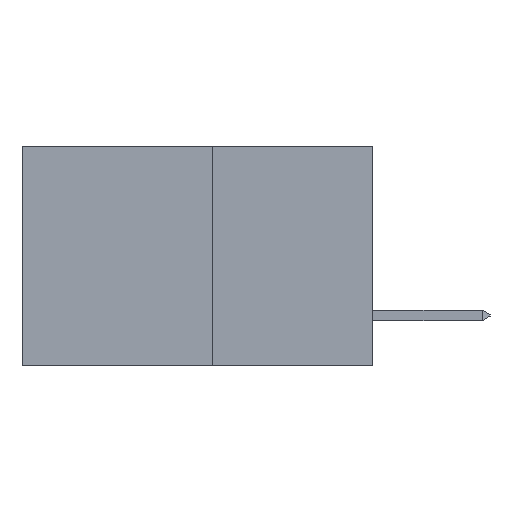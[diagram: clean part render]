
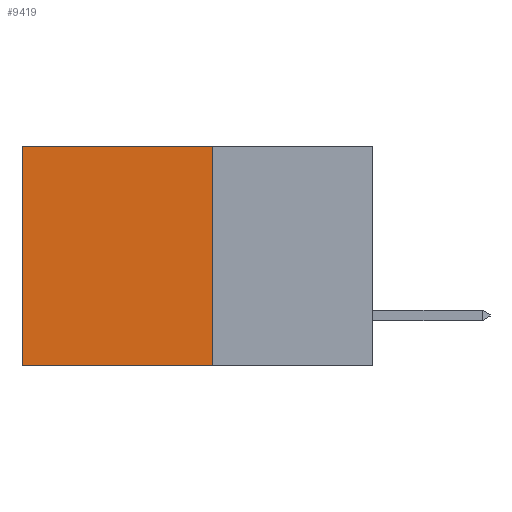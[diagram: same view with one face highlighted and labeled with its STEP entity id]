
A CAD part, left-side view. The second image highlights one B-rep face of the part: STEP entity #9419.
In plain terms, the highlighted planar face has unit normal (-1, 0, 0).
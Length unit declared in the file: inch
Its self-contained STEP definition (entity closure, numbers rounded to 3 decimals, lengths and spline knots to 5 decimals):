
#401 = CARTESIAN_POINT ( 'NONE',  ( 0.277, 0.27, -0.37 ) ) ;
#2085 = LINE ( 'NONE', #2932, #7066 ) ;
#2596 = FACE_OUTER_BOUND ( 'NONE', #20494, .T. ) ;
#2932 = CARTESIAN_POINT ( 'NONE',  ( 0.277, 0.59, -0.37 ) ) ;
#2999 = EDGE_CURVE ( 'NONE', #23021, #4360, #23911, .T. ) ;
#3555 = VERTEX_POINT ( 'NONE', #27264 ) ;
#3625 = ORIENTED_EDGE ( 'NONE', *, *, #11713, .T. ) ;
#4360 = VERTEX_POINT ( 'NONE', #6906 ) ;
#4636 = CARTESIAN_POINT ( 'NONE',  ( 0.277, 0.27, 0. ) ) ;
#6606 = DIRECTION ( 'NONE',  ( 0., 0., -1. ) ) ;
#6906 = CARTESIAN_POINT ( 'NONE',  ( 0.277, 0.59, -0.37 ) ) ;
#7066 = VECTOR ( 'NONE', #19812, 39.37008 ) ;
#8516 = LINE ( 'NONE', #4636, #23978 ) ;
#8919 = AXIS2_PLACEMENT_3D ( 'NONE', #22892, #24997, #12374 ) ;
#9419 = ADVANCED_FACE ( 'NONE', ( #2596 ), #20696, .F. ) ;
#10363 = ORIENTED_EDGE ( 'NONE', *, *, #2999, .F. ) ;
#11713 = EDGE_CURVE ( 'NONE', #17620, #4360, #2085, .T. ) ;
#12374 = DIRECTION ( 'NONE',  ( 0., 0., -1. ) ) ;
#14006 = EDGE_CURVE ( 'NONE', #3555, #23021, #16398, .T. ) ;
#14808 = EDGE_CURVE ( 'NONE', #3555, #17620, #8516, .T. ) ;
#15426 = DIRECTION ( 'NONE',  ( 0., 1., 0. ) ) ;
#15785 = ORIENTED_EDGE ( 'NONE', *, *, #14006, .F. ) ;
#16398 = LINE ( 'NONE', #17052, #26978 ) ;
#17052 = CARTESIAN_POINT ( 'NONE',  ( 0.277, 0.27, -0.37 ) ) ;
#17620 = VERTEX_POINT ( 'NONE', #26310 ) ;
#18315 = VECTOR ( 'NONE', #15426, 39.37008 ) ;
#19812 = DIRECTION ( 'NONE',  ( 0., 0., -1. ) ) ;
#20494 = EDGE_LOOP ( 'NONE', ( #3625, #10363, #15785, #22190 ) ) ;
#20696 = PLANE ( 'NONE',  #8919 ) ;
#22190 = ORIENTED_EDGE ( 'NONE', *, *, #14808, .T. ) ;
#22892 = CARTESIAN_POINT ( 'NONE',  ( 0.277, 0.27, -0.37 ) ) ;
#23021 = VERTEX_POINT ( 'NONE', #401 ) ;
#23593 = DIRECTION ( 'NONE',  ( 0., 1., 0. ) ) ;
#23911 = LINE ( 'NONE', #26055, #18315 ) ;
#23978 = VECTOR ( 'NONE', #23593, 39.37008 ) ;
#24997 = DIRECTION ( 'NONE',  ( 1., 0., 0. ) ) ;
#26055 = CARTESIAN_POINT ( 'NONE',  ( 0.277, 0.27, -0.37 ) ) ;
#26310 = CARTESIAN_POINT ( 'NONE',  ( 0.277, 0.59, 0. ) ) ;
#26978 = VECTOR ( 'NONE', #6606, 39.37008 ) ;
#27264 = CARTESIAN_POINT ( 'NONE',  ( 0.277, 0.27, 0. ) ) ;
